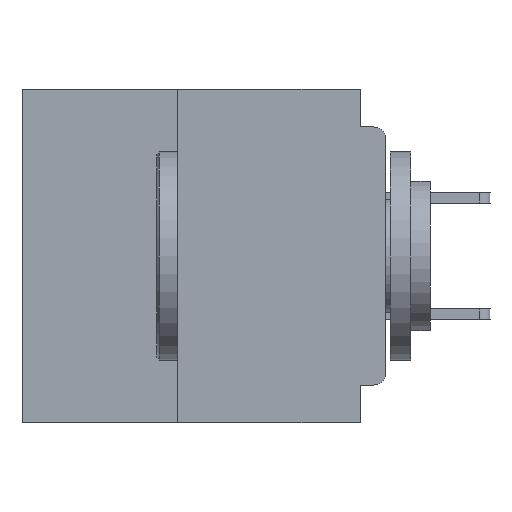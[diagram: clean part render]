
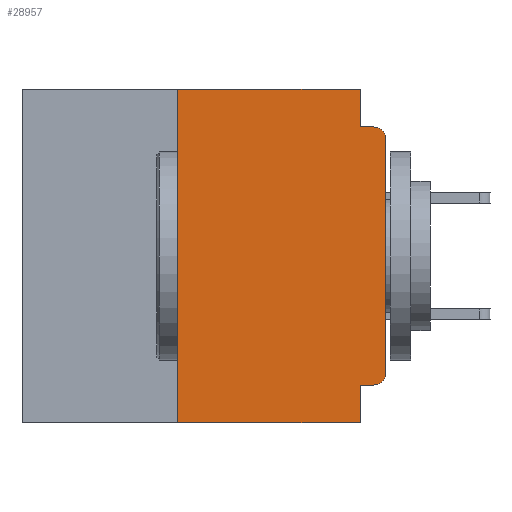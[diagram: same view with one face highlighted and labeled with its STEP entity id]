
A CAD part, left-side view. The second image highlights one B-rep face of the part: STEP entity #28957.
In plain terms, the highlighted planar face has unit normal (-1, 0, 0).
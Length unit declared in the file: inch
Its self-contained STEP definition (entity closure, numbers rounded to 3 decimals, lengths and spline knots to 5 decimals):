
#767 = CARTESIAN_POINT ( 'NONE',  ( 0., 0., -0.06 ) ) ;
#1794 = LINE ( 'NONE', #34709, #50902 ) ;
#3009 = ORIENTED_EDGE ( 'NONE', *, *, #40982, .T. ) ;
#4086 = DIRECTION ( 'NONE',  ( 0., 0., -1. ) ) ;
#4087 = VECTOR ( 'NONE', #28065, 39.37008 ) ;
#4584 = CARTESIAN_POINT ( 'NONE',  ( 0., 0.015, -0.34 ) ) ;
#4841 = DIRECTION ( 'NONE',  ( 0., -1., 0. ) ) ;
#5165 = CARTESIAN_POINT ( 'NONE',  ( 0., 0.437, 0. ) ) ;
#6503 = AXIS2_PLACEMENT_3D ( 'NONE', #5165, #33606, #48011 ) ;
#6718 = CARTESIAN_POINT ( 'NONE',  ( 0., 0.015, -0.06 ) ) ;
#7767 = LINE ( 'NONE', #61272, #44236 ) ;
#7792 = AXIS2_PLACEMENT_3D ( 'NONE', #6718, #39975, #11492 ) ;
#8213 = EDGE_CURVE ( 'NONE', #29205, #58673, #7767, .T. ) ;
#8870 = DIRECTION ( 'NONE',  ( 0., 0., 1. ) ) ;
#9246 = LINE ( 'NONE', #9640, #56851 ) ;
#9294 = ORIENTED_EDGE ( 'NONE', *, *, #53111, .F. ) ;
#9342 = DIRECTION ( 'NONE',  ( 0., 0., -1. ) ) ;
#9640 = CARTESIAN_POINT ( 'NONE',  ( 0., 0.437, -0.4 ) ) ;
#11492 = DIRECTION ( 'NONE',  ( 0., 0., -1. ) ) ;
#11689 = ORIENTED_EDGE ( 'NONE', *, *, #56942, .T. ) ;
#12375 = LINE ( 'NONE', #28420, #23496 ) ;
#14071 = AXIS2_PLACEMENT_3D ( 'NONE', #4584, #37820, #9342 ) ;
#14330 = VERTEX_POINT ( 'NONE', #20015 ) ;
#14678 = EDGE_CURVE ( 'NONE', #14330, #17545, #34040, .T. ) ;
#15327 = ORIENTED_EDGE ( 'NONE', *, *, #14678, .F. ) ;
#17545 = VERTEX_POINT ( 'NONE', #31578 ) ;
#18383 = CARTESIAN_POINT ( 'NONE',  ( 0., 0.015, -0.045 ) ) ;
#18850 = ORIENTED_EDGE ( 'NONE', *, *, #37901, .F. ) ;
#19043 = VERTEX_POINT ( 'NONE', #18383 ) ;
#20015 = CARTESIAN_POINT ( 'NONE',  ( 0., 0.25, -0.4 ) ) ;
#20118 = CARTESIAN_POINT ( 'NONE',  ( 0., 0.031, -0.4 ) ) ;
#20233 = ORIENTED_EDGE ( 'NONE', *, *, #8213, .T. ) ;
#20564 = DIRECTION ( 'NONE',  ( 0., -1., 0. ) ) ;
#21094 = CIRCLE ( 'NONE', #7792, 0.015 ) ;
#21723 = VERTEX_POINT ( 'NONE', #49870 ) ;
#23496 = VECTOR ( 'NONE', #4841, 39.37008 ) ;
#24477 = CARTESIAN_POINT ( 'NONE',  ( 0., 0.031, -0.355 ) ) ;
#27587 = CARTESIAN_POINT ( 'NONE',  ( 0., 0.25, -0.4 ) ) ;
#28011 = LINE ( 'NONE', #56181, #40742 ) ;
#28065 = DIRECTION ( 'NONE',  ( 0., 1., 0. ) ) ;
#28420 = CARTESIAN_POINT ( 'NONE',  ( 0., 0., -0.045 ) ) ;
#28957 = ADVANCED_FACE ( 'NONE', ( #34028 ), #43225, .F. ) ;
#29205 = VERTEX_POINT ( 'NONE', #44858 ) ;
#30201 = EDGE_CURVE ( 'NONE', #21723, #19043, #12375, .T. ) ;
#31471 = EDGE_CURVE ( 'NONE', #55606, #59830, #56123, .T. ) ;
#31578 = CARTESIAN_POINT ( 'NONE',  ( 0., 0.25, 0. ) ) ;
#33127 = ORIENTED_EDGE ( 'NONE', *, *, #30201, .F. ) ;
#33606 = DIRECTION ( 'NONE',  ( 1., 0., 0. ) ) ;
#33741 = VECTOR ( 'NONE', #4086, 39.37008 ) ;
#34028 = FACE_OUTER_BOUND ( 'NONE', #43252, .T. ) ;
#34040 = LINE ( 'NONE', #27587, #59341 ) ;
#34709 = CARTESIAN_POINT ( 'NONE',  ( 0., 0.437, 0. ) ) ;
#35796 = CIRCLE ( 'NONE', #14071, 0.015 ) ;
#37820 = DIRECTION ( 'NONE',  ( -1., 0., 0. ) ) ;
#37901 = EDGE_CURVE ( 'NONE', #17545, #49648, #1794, .T. ) ;
#38160 = DIRECTION ( 'NONE',  ( 0., -1., 0. ) ) ;
#39072 = CARTESIAN_POINT ( 'NONE',  ( 0., 0.031, 0. ) ) ;
#39975 = DIRECTION ( 'NONE',  ( -1., 0., 0. ) ) ;
#40738 = EDGE_CURVE ( 'NONE', #14330, #43419, #9246, .T. ) ;
#40742 = VECTOR ( 'NONE', #60937, 39.37008 ) ;
#40982 = EDGE_CURVE ( 'NONE', #58673, #19043, #21094, .T. ) ;
#41826 = ORIENTED_EDGE ( 'NONE', *, *, #44065, .F. ) ;
#43225 = PLANE ( 'NONE',  #6503 ) ;
#43252 = EDGE_LOOP ( 'NONE', ( #20233, #3009, #33127, #41826, #18850, #15327, #46172, #9294, #51917, #11689 ) ) ;
#43419 = VERTEX_POINT ( 'NONE', #20118 ) ;
#44065 = EDGE_CURVE ( 'NONE', #49648, #21723, #59050, .T. ) ;
#44236 = VECTOR ( 'NONE', #8870, 39.37008 ) ;
#44858 = CARTESIAN_POINT ( 'NONE',  ( 0., 0., -0.34 ) ) ;
#46172 = ORIENTED_EDGE ( 'NONE', *, *, #40738, .T. ) ;
#46536 = CARTESIAN_POINT ( 'NONE',  ( 0., 0.015, -0.355 ) ) ;
#48011 = DIRECTION ( 'NONE',  ( 0., 0., -1. ) ) ;
#49648 = VERTEX_POINT ( 'NONE', #39072 ) ;
#49870 = CARTESIAN_POINT ( 'NONE',  ( 0., 0.031, -0.045 ) ) ;
#50902 = VECTOR ( 'NONE', #20564, 39.37008 ) ;
#51917 = ORIENTED_EDGE ( 'NONE', *, *, #31471, .F. ) ;
#53111 = EDGE_CURVE ( 'NONE', #59830, #43419, #28011, .T. ) ;
#55606 = VERTEX_POINT ( 'NONE', #46536 ) ;
#56123 = LINE ( 'NONE', #61416, #4087 ) ;
#56181 = CARTESIAN_POINT ( 'NONE',  ( 0., 0.031, -0.4 ) ) ;
#56851 = VECTOR ( 'NONE', #38160, 39.37008 ) ;
#56942 = EDGE_CURVE ( 'NONE', #55606, #29205, #35796, .T. ) ;
#58673 = VERTEX_POINT ( 'NONE', #767 ) ;
#59050 = LINE ( 'NONE', #60990, #33741 ) ;
#59341 = VECTOR ( 'NONE', #60931, 39.37008 ) ;
#59830 = VERTEX_POINT ( 'NONE', #24477 ) ;
#60931 = DIRECTION ( 'NONE',  ( 0., 0., 1. ) ) ;
#60937 = DIRECTION ( 'NONE',  ( 0., 0., -1. ) ) ;
#60990 = CARTESIAN_POINT ( 'NONE',  ( 0., 0.031, 0. ) ) ;
#61272 = CARTESIAN_POINT ( 'NONE',  ( 0., 0., 0. ) ) ;
#61416 = CARTESIAN_POINT ( 'NONE',  ( 0., 0., -0.355 ) ) ;
